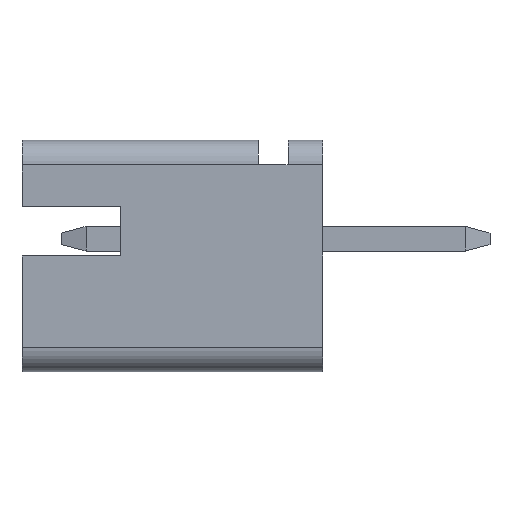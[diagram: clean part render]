
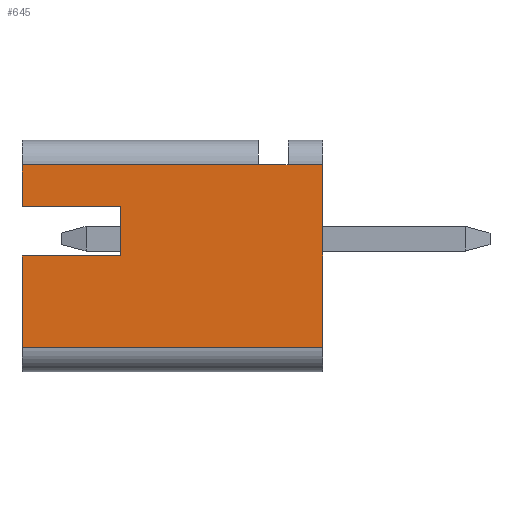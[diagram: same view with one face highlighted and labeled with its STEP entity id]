
A CAD part, left-side view. The second image highlights one B-rep face of the part: STEP entity #645.
In plain terms, the highlighted planar face has unit normal (-1, 0, 0).
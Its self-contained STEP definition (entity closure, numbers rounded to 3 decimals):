
#29 = LINE ( 'NONE', #999, #1286 ) ;
#48 = EDGE_CURVE ( 'NONE', #1033, #2106, #566, .T. ) ;
#71 = CARTESIAN_POINT ( 'NONE',  ( -2., 0., 1.5 ) ) ;
#101 = VERTEX_POINT ( 'NONE', #1755 ) ;
#104 = CARTESIAN_POINT ( 'NONE',  ( -2., 6.1, 1.5 ) ) ;
#114 = PLANE ( 'NONE',  #2260 ) ;
#119 = CARTESIAN_POINT ( 'NONE',  ( -2., 6.1, 0.65 ) ) ;
#177 = DIRECTION ( 'NONE',  ( 0., 1., 0. ) ) ;
#184 = VECTOR ( 'NONE', #483, 1000. ) ;
#228 = VERTEX_POINT ( 'NONE', #2249 ) ;
#325 = DIRECTION ( 'NONE',  ( 0., 0., 1. ) ) ;
#357 = DIRECTION ( 'NONE',  ( 0., 0., -1. ) ) ;
#428 = EDGE_CURVE ( 'NONE', #101, #642, #965, .T. ) ;
#448 = CARTESIAN_POINT ( 'NONE',  ( -2., 4.1, 0.65 ) ) ;
#468 = LINE ( 'NONE', #1253, #184 ) ;
#470 = CARTESIAN_POINT ( 'NONE',  ( -2., 6.1, -0.35 ) ) ;
#471 = VECTOR ( 'NONE', #325, 1000. ) ;
#476 = LINE ( 'NONE', #711, #1990 ) ;
#483 = DIRECTION ( 'NONE',  ( 0., 0., 1. ) ) ;
#505 = ORIENTED_EDGE ( 'NONE', *, *, #2247, .F. ) ;
#553 = VECTOR ( 'NONE', #1870, 1000. ) ;
#566 = LINE ( 'NONE', #1393, #1306 ) ;
#591 = EDGE_CURVE ( 'NONE', #717, #1033, #29, .T. ) ;
#642 = VERTEX_POINT ( 'NONE', #1458 ) ;
#645 = ADVANCED_FACE ( 'NONE', ( #2238 ), #114, .F. ) ;
#658 = ORIENTED_EDGE ( 'NONE', *, *, #48, .F. ) ;
#695 = VERTEX_POINT ( 'NONE', #1667 ) ;
#711 = CARTESIAN_POINT ( 'NONE',  ( -2., 0., 1.5 ) ) ;
#717 = VERTEX_POINT ( 'NONE', #470 ) ;
#726 = CARTESIAN_POINT ( 'NONE',  ( -2., 6.1, 0.65 ) ) ;
#772 = CARTESIAN_POINT ( 'NONE',  ( -2., 0., 2. ) ) ;
#930 = VERTEX_POINT ( 'NONE', #1492 ) ;
#952 = EDGE_CURVE ( 'NONE', #228, #1771, #476, .T. ) ;
#965 = LINE ( 'NONE', #772, #2075 ) ;
#969 = VECTOR ( 'NONE', #177, 1000. ) ;
#999 = CARTESIAN_POINT ( 'NONE',  ( -2., 6.1, -0.35 ) ) ;
#1033 = VERTEX_POINT ( 'NONE', #1544 ) ;
#1072 = CARTESIAN_POINT ( 'NONE',  ( -2., 6.1, -0.35 ) ) ;
#1075 = VERTEX_POINT ( 'NONE', #726 ) ;
#1082 = CARTESIAN_POINT ( 'NONE',  ( -2., 0., -2.2 ) ) ;
#1098 = LINE ( 'NONE', #1082, #1738 ) ;
#1106 = ORIENTED_EDGE ( 'NONE', *, *, #2534, .F. ) ;
#1171 = DIRECTION ( 'NONE',  ( 0., -1., 0. ) ) ;
#1191 = EDGE_LOOP ( 'NONE', ( #1106, #1298, #2239, #2004, #2256, #1578, #1799, #505, #658, #1264 ) ) ;
#1253 = CARTESIAN_POINT ( 'NONE',  ( -2., 6.1, 2. ) ) ;
#1264 = ORIENTED_EDGE ( 'NONE', *, *, #591, .F. ) ;
#1286 = VECTOR ( 'NONE', #1171, 1000. ) ;
#1298 = ORIENTED_EDGE ( 'NONE', *, *, #2097, .T. ) ;
#1306 = VECTOR ( 'NONE', #1349, 1000. ) ;
#1349 = DIRECTION ( 'NONE',  ( 0., 0., 1. ) ) ;
#1354 = CARTESIAN_POINT ( 'NONE',  ( -2., 1.3, 1.5 ) ) ;
#1361 = EDGE_CURVE ( 'NONE', #1075, #1771, #468, .T. ) ;
#1393 = CARTESIAN_POINT ( 'NONE',  ( -2., 4.1, 0.65 ) ) ;
#1458 = CARTESIAN_POINT ( 'NONE',  ( -2., 0., -2.2 ) ) ;
#1478 = DIRECTION ( 'NONE',  ( 0., 1., 0. ) ) ;
#1492 = CARTESIAN_POINT ( 'NONE',  ( -2., 6.1, -2.2 ) ) ;
#1544 = CARTESIAN_POINT ( 'NONE',  ( -2., 4.1, -0.35 ) ) ;
#1578 = ORIENTED_EDGE ( 'NONE', *, *, #952, .T. ) ;
#1615 = EDGE_CURVE ( 'NONE', #101, #695, #1826, .T. ) ;
#1667 = CARTESIAN_POINT ( 'NONE',  ( -2., 0.7, 1.5 ) ) ;
#1687 = DIRECTION ( 'NONE',  ( 0., -1., 0. ) ) ;
#1738 = VECTOR ( 'NONE', #1687, 1000. ) ;
#1755 = CARTESIAN_POINT ( 'NONE',  ( -2., 0., 1.5 ) ) ;
#1769 = LINE ( 'NONE', #1354, #2385 ) ;
#1771 = VERTEX_POINT ( 'NONE', #104 ) ;
#1799 = ORIENTED_EDGE ( 'NONE', *, *, #1361, .F. ) ;
#1823 = DIRECTION ( 'NONE',  ( 0., 0., -1. ) ) ;
#1826 = LINE ( 'NONE', #71, #553 ) ;
#1870 = DIRECTION ( 'NONE',  ( 0., 1., 0. ) ) ;
#1944 = LINE ( 'NONE', #119, #969 ) ;
#1990 = VECTOR ( 'NONE', #1478, 1000. ) ;
#2004 = ORIENTED_EDGE ( 'NONE', *, *, #1615, .T. ) ;
#2047 = DIRECTION ( 'NONE',  ( 1., 0., 0. ) ) ;
#2062 = CARTESIAN_POINT ( 'NONE',  ( -2., 0., 0. ) ) ;
#2075 = VECTOR ( 'NONE', #357, 1000. ) ;
#2090 = LINE ( 'NONE', #1072, #471 ) ;
#2097 = EDGE_CURVE ( 'NONE', #930, #642, #1098, .T. ) ;
#2106 = VERTEX_POINT ( 'NONE', #448 ) ;
#2132 = DIRECTION ( 'NONE',  ( 0., -1., 0. ) ) ;
#2171 = EDGE_CURVE ( 'NONE', #228, #695, #1769, .T. ) ;
#2238 = FACE_OUTER_BOUND ( 'NONE', #1191, .T. ) ;
#2239 = ORIENTED_EDGE ( 'NONE', *, *, #428, .F. ) ;
#2247 = EDGE_CURVE ( 'NONE', #2106, #1075, #1944, .T. ) ;
#2249 = CARTESIAN_POINT ( 'NONE',  ( -2., 1.3, 1.5 ) ) ;
#2256 = ORIENTED_EDGE ( 'NONE', *, *, #2171, .F. ) ;
#2260 = AXIS2_PLACEMENT_3D ( 'NONE', #2062, #2047, #1823 ) ;
#2385 = VECTOR ( 'NONE', #2132, 1000. ) ;
#2534 = EDGE_CURVE ( 'NONE', #930, #717, #2090, .T. ) ;
